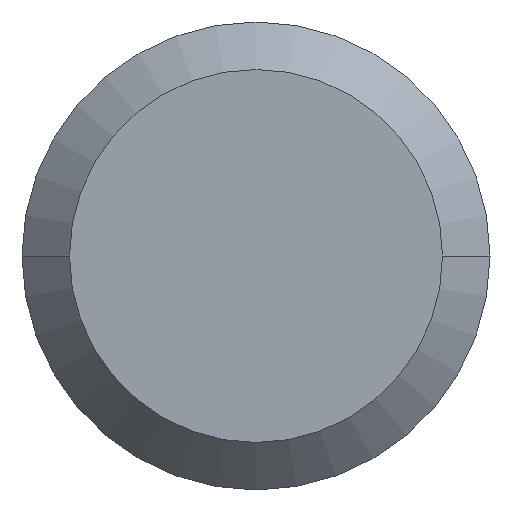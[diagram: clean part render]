
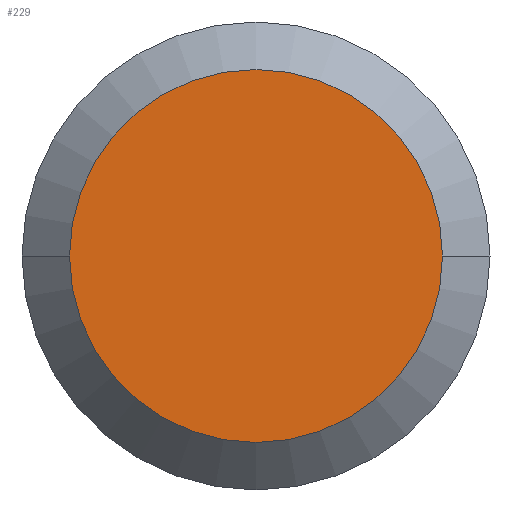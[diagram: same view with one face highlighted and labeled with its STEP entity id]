
A CAD part, left-side view. The second image highlights one B-rep face of the part: STEP entity #229.
In plain terms, the highlighted planar face has unit normal (-1, 0, 0).
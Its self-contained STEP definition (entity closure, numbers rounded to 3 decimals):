
#25 = CARTESIAN_POINT ( 'NONE',  ( -11.443, -1.994, 0. ) ) ;
#32 = ORIENTED_EDGE ( 'NONE', *, *, #362, .F. ) ;
#48 = FACE_OUTER_BOUND ( 'NONE', #242, .T. ) ;
#79 = DIRECTION ( 'NONE',  ( 0., 0., 1. ) ) ;
#83 = CIRCLE ( 'NONE', #330, 1.994 ) ;
#115 = ORIENTED_EDGE ( 'NONE', *, *, #278, .F. ) ;
#116 = CIRCLE ( 'NONE', #357, 1.994 ) ;
#130 = CARTESIAN_POINT ( 'NONE',  ( -11.443, 0., 0. ) ) ;
#175 = CARTESIAN_POINT ( 'NONE',  ( -11.443, 0., 0. ) ) ;
#192 = VERTEX_POINT ( 'NONE', #25 ) ;
#193 = PLANE ( 'NONE',  #382 ) ;
#196 = DIRECTION ( 'NONE',  ( 1., 0., 0. ) ) ;
#216 = VERTEX_POINT ( 'NONE', #460 ) ;
#220 = DIRECTION ( 'NONE',  ( 0., -1., 0. ) ) ;
#229 = ADVANCED_FACE ( 'NONE', ( #48 ), #193, .T. ) ;
#242 = EDGE_LOOP ( 'NONE', ( #32, #115 ) ) ;
#278 = EDGE_CURVE ( 'NONE', #216, #192, #116, .T. ) ;
#330 = AXIS2_PLACEMENT_3D ( 'NONE', #130, #429, #220 ) ;
#357 = AXIS2_PLACEMENT_3D ( 'NONE', #175, #196, #403 ) ;
#358 = CARTESIAN_POINT ( 'NONE',  ( -11.443, 2.502, 0. ) ) ;
#362 = EDGE_CURVE ( 'NONE', #192, #216, #83, .T. ) ;
#380 = DIRECTION ( 'NONE',  ( -1., 0., 0. ) ) ;
#382 = AXIS2_PLACEMENT_3D ( 'NONE', #358, #380, #79 ) ;
#403 = DIRECTION ( 'NONE',  ( 0., -1., 0. ) ) ;
#429 = DIRECTION ( 'NONE',  ( 1., 0., 0. ) ) ;
#460 = CARTESIAN_POINT ( 'NONE',  ( -11.443, 1.994, 0. ) ) ;
